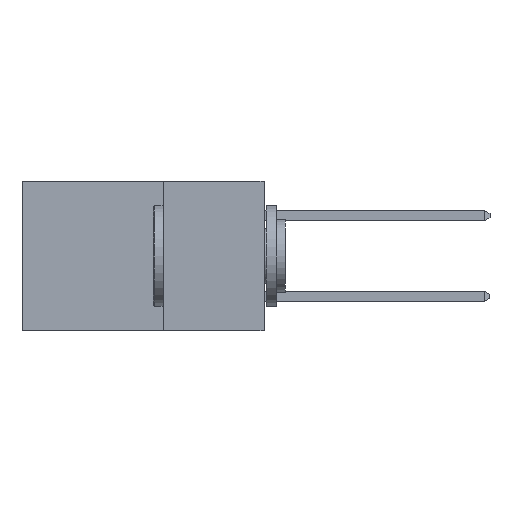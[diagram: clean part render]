
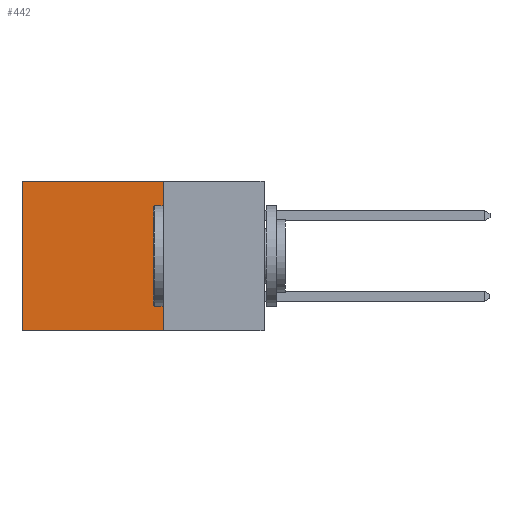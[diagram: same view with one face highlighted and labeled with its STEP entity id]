
A CAD part, left-side view. The second image highlights one B-rep face of the part: STEP entity #442.
In plain terms, the highlighted planar face has unit normal (-1, 0, 0).
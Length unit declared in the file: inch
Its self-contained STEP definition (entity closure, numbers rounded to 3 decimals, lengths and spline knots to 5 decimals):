
#381 = AXIS2_PLACEMENT_3D ( 'NONE', #6565, #1807, #7327 ) ;
#442 = ADVANCED_FACE ( 'NONE', ( #6459 ), #4166, .F. ) ;
#591 = DIRECTION ( 'NONE',  ( 0., 0., -1. ) ) ;
#709 = DIRECTION ( 'NONE',  ( 0., 0., -1. ) ) ;
#1403 = CARTESIAN_POINT ( 'NONE',  ( 0.2615, 0.25, -0.37 ) ) ;
#1807 = DIRECTION ( 'NONE',  ( 1., 0., 0. ) ) ;
#2379 = CARTESIAN_POINT ( 'NONE',  ( 0.2615, 0.6, -0.37 ) ) ;
#2923 = CARTESIAN_POINT ( 'NONE',  ( 0.2615, 0.25, 0. ) ) ;
#2997 = ORIENTED_EDGE ( 'NONE', *, *, #8713, .F. ) ;
#3732 = EDGE_CURVE ( 'NONE', #6557, #5456, #7678, .T. ) ;
#4166 = PLANE ( 'NONE',  #381 ) ;
#4378 = VECTOR ( 'NONE', #591, 39.37008 ) ;
#4987 = CARTESIAN_POINT ( 'NONE',  ( 0.2615, 0.25, 0. ) ) ;
#5081 = EDGE_LOOP ( 'NONE', ( #6462, #7905, #2997, #6892 ) ) ;
#5192 = VECTOR ( 'NONE', #8543, 39.37008 ) ;
#5328 = CARTESIAN_POINT ( 'NONE',  ( 0.2615, 0.25, -0.37 ) ) ;
#5344 = LINE ( 'NONE', #2379, #6716 ) ;
#5362 = DIRECTION ( 'NONE',  ( 0., 1., 0. ) ) ;
#5410 = EDGE_CURVE ( 'NONE', #7320, #8409, #10198, .T. ) ;
#5456 = VERTEX_POINT ( 'NONE', #7055 ) ;
#6459 = FACE_OUTER_BOUND ( 'NONE', #5081, .T. ) ;
#6462 = ORIENTED_EDGE ( 'NONE', *, *, #8269, .T. ) ;
#6557 = VERTEX_POINT ( 'NONE', #4987 ) ;
#6565 = CARTESIAN_POINT ( 'NONE',  ( 0.2615, 0.25, -0.37 ) ) ;
#6588 = CARTESIAN_POINT ( 'NONE',  ( 0.2615, 0.6, -0.37 ) ) ;
#6716 = VECTOR ( 'NONE', #709, 39.37008 ) ;
#6892 = ORIENTED_EDGE ( 'NONE', *, *, #3732, .T. ) ;
#7055 = CARTESIAN_POINT ( 'NONE',  ( 0.2615, 0.6, 0. ) ) ;
#7097 = LINE ( 'NONE', #5328, #4378 ) ;
#7311 = VECTOR ( 'NONE', #5362, 39.37008 ) ;
#7320 = VERTEX_POINT ( 'NONE', #1403 ) ;
#7327 = DIRECTION ( 'NONE',  ( 0., 0., -1. ) ) ;
#7651 = CARTESIAN_POINT ( 'NONE',  ( 0.2615, 0.25, -0.37 ) ) ;
#7678 = LINE ( 'NONE', #2923, #7311 ) ;
#7905 = ORIENTED_EDGE ( 'NONE', *, *, #5410, .F. ) ;
#8269 = EDGE_CURVE ( 'NONE', #5456, #8409, #5344, .T. ) ;
#8409 = VERTEX_POINT ( 'NONE', #6588 ) ;
#8543 = DIRECTION ( 'NONE',  ( 0., 1., 0. ) ) ;
#8713 = EDGE_CURVE ( 'NONE', #6557, #7320, #7097, .T. ) ;
#10198 = LINE ( 'NONE', #7651, #5192 ) ;
